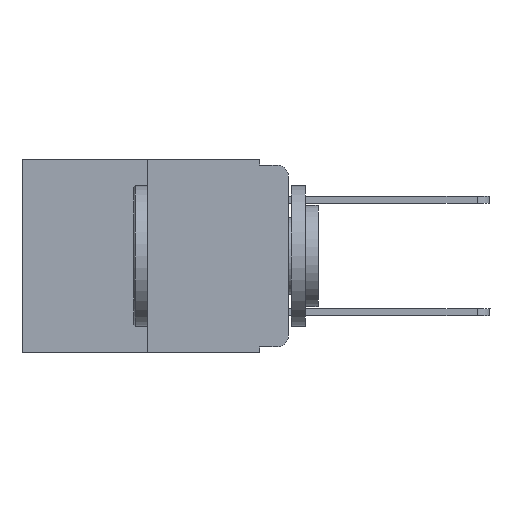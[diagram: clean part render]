
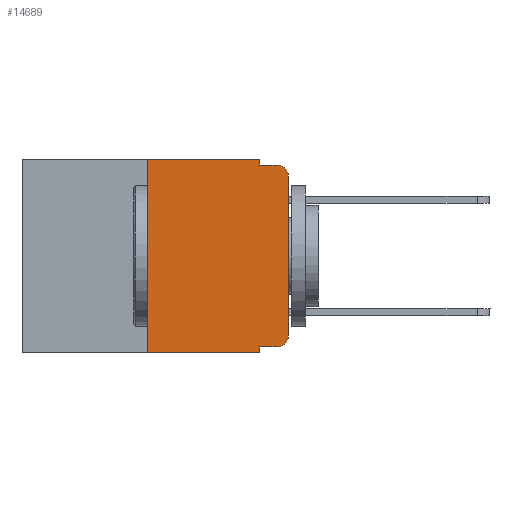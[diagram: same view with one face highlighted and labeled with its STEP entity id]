
A CAD part, left-side view. The second image highlights one B-rep face of the part: STEP entity #14689.
In plain terms, the highlighted planar face has unit normal (-1, 0, 0).
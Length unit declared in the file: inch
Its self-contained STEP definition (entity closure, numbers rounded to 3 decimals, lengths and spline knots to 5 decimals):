
#110 = DIRECTION ( 'NONE',  ( -1., 0., 0. ) ) ;
#189 = CARTESIAN_POINT ( 'NONE',  ( 0., 0.25, 0. ) ) ;
#237 = CARTESIAN_POINT ( 'NONE',  ( 0., 0.051, -0.333 ) ) ;
#295 = CARTESIAN_POINT ( 'NONE',  ( 0., 0.051, 0. ) ) ;
#404 = EDGE_CURVE ( 'NONE', #11798, #13101, #13912, .T. ) ;
#758 = ORIENTED_EDGE ( 'NONE', *, *, #7541, .T. ) ;
#784 = EDGE_CURVE ( 'NONE', #2574, #2361, #12662, .T. ) ;
#806 = EDGE_CURVE ( 'NONE', #6887, #14524, #15415, .T. ) ;
#812 = CARTESIAN_POINT ( 'NONE',  ( 0., 0., -0.313 ) ) ;
#875 = CARTESIAN_POINT ( 'NONE',  ( 0., 0., -0.03 ) ) ;
#1361 = EDGE_CURVE ( 'NONE', #11770, #13101, #15716, .T. ) ;
#1905 = ORIENTED_EDGE ( 'NONE', *, *, #8811, .F. ) ;
#1997 = CARTESIAN_POINT ( 'NONE',  ( 0., 0.473, -0.343 ) ) ;
#2109 = ORIENTED_EDGE ( 'NONE', *, *, #1361, .T. ) ;
#2127 = CARTESIAN_POINT ( 'NONE',  ( 0., 0.051, -0.333 ) ) ;
#2243 = LINE ( 'NONE', #4614, #11854 ) ;
#2361 = VERTEX_POINT ( 'NONE', #9852 ) ;
#2376 = CARTESIAN_POINT ( 'NONE',  ( 0., 0.051, 0. ) ) ;
#2535 = LINE ( 'NONE', #5153, #6289 ) ;
#2574 = VERTEX_POINT ( 'NONE', #189 ) ;
#2755 = DIRECTION ( 'NONE',  ( 0., -1., 0. ) ) ;
#2817 = DIRECTION ( 'NONE',  ( 0., 0., 1. ) ) ;
#2973 = AXIS2_PLACEMENT_3D ( 'NONE', #4204, #4367, #7921 ) ;
#3584 = LINE ( 'NONE', #2376, #13242 ) ;
#3916 = DIRECTION ( 'NONE',  ( 0., 0., -1. ) ) ;
#4102 = VECTOR ( 'NONE', #2755, 39.37008 ) ;
#4137 = VECTOR ( 'NONE', #5857, 39.37008 ) ;
#4204 = CARTESIAN_POINT ( 'NONE',  ( 0., 0.473, 0. ) ) ;
#4269 = CARTESIAN_POINT ( 'NONE',  ( 0., 0.051, -0.343 ) ) ;
#4367 = DIRECTION ( 'NONE',  ( 1., 0., 0. ) ) ;
#4370 = CIRCLE ( 'NONE', #14857, 0.02 ) ;
#4614 = CARTESIAN_POINT ( 'NONE',  ( 0., 0.051, -0.01 ) ) ;
#5028 = EDGE_CURVE ( 'NONE', #11826, #7764, #2243, .T. ) ;
#5089 = CARTESIAN_POINT ( 'NONE',  ( 0., 0.02, -0.03 ) ) ;
#5135 = LINE ( 'NONE', #237, #4102 ) ;
#5153 = CARTESIAN_POINT ( 'NONE',  ( 0., 0., 0. ) ) ;
#5310 = DIRECTION ( 'NONE',  ( 0., 0., 1. ) ) ;
#5428 = DIRECTION ( 'NONE',  ( 0., 0., -1. ) ) ;
#5498 = CARTESIAN_POINT ( 'NONE',  ( 0., 0.051, -0.01 ) ) ;
#5857 = DIRECTION ( 'NONE',  ( 0., -1., 0. ) ) ;
#6289 = VECTOR ( 'NONE', #5310, 39.37008 ) ;
#6387 = ORIENTED_EDGE ( 'NONE', *, *, #404, .F. ) ;
#6408 = ORIENTED_EDGE ( 'NONE', *, *, #15107, .F. ) ;
#6887 = VERTEX_POINT ( 'NONE', #7319 ) ;
#6968 = EDGE_CURVE ( 'NONE', #12727, #7764, #4370, .T. ) ;
#7319 = CARTESIAN_POINT ( 'NONE',  ( 0., 0.02, -0.333 ) ) ;
#7366 = CARTESIAN_POINT ( 'NONE',  ( 0., 0.02, -0.01 ) ) ;
#7541 = EDGE_CURVE ( 'NONE', #14524, #12727, #2535, .T. ) ;
#7764 = VERTEX_POINT ( 'NONE', #7366 ) ;
#7921 = DIRECTION ( 'NONE',  ( 0., 0., -1. ) ) ;
#8022 = CARTESIAN_POINT ( 'NONE',  ( 0., 0.02, -0.313 ) ) ;
#8543 = ORIENTED_EDGE ( 'NONE', *, *, #6968, .T. ) ;
#8811 = EDGE_CURVE ( 'NONE', #2361, #11826, #3584, .T. ) ;
#9339 = CARTESIAN_POINT ( 'NONE',  ( 0., 0.473, 0. ) ) ;
#9404 = FACE_OUTER_BOUND ( 'NONE', #14878, .T. ) ;
#9462 = EDGE_CURVE ( 'NONE', #11798, #6887, #5135, .T. ) ;
#9852 = CARTESIAN_POINT ( 'NONE',  ( 0., 0.051, 0. ) ) ;
#10184 = VECTOR ( 'NONE', #10565, 39.37008 ) ;
#10424 = AXIS2_PLACEMENT_3D ( 'NONE', #8022, #14267, #13971 ) ;
#10565 = DIRECTION ( 'NONE',  ( 0., -1., 0. ) ) ;
#11770 = VERTEX_POINT ( 'NONE', #11834 ) ;
#11798 = VERTEX_POINT ( 'NONE', #2127 ) ;
#11826 = VERTEX_POINT ( 'NONE', #5498 ) ;
#11834 = CARTESIAN_POINT ( 'NONE',  ( 0., 0.25, -0.343 ) ) ;
#11854 = VECTOR ( 'NONE', #13331, 39.37008 ) ;
#12662 = LINE ( 'NONE', #9339, #10184 ) ;
#12704 = VECTOR ( 'NONE', #2817, 39.37008 ) ;
#12727 = VERTEX_POINT ( 'NONE', #875 ) ;
#13101 = VERTEX_POINT ( 'NONE', #4269 ) ;
#13242 = VECTOR ( 'NONE', #3916, 39.37008 ) ;
#13331 = DIRECTION ( 'NONE',  ( 0., -1., 0. ) ) ;
#13912 = LINE ( 'NONE', #295, #15915 ) ;
#13954 = ORIENTED_EDGE ( 'NONE', *, *, #9462, .T. ) ;
#13968 = DIRECTION ( 'NONE',  ( 0., 0., -1. ) ) ;
#13971 = DIRECTION ( 'NONE',  ( 0., 0., -1. ) ) ;
#14144 = CARTESIAN_POINT ( 'NONE',  ( 0., 0.25, 0. ) ) ;
#14267 = DIRECTION ( 'NONE',  ( -1., 0., 0. ) ) ;
#14524 = VERTEX_POINT ( 'NONE', #812 ) ;
#14689 = ADVANCED_FACE ( 'NONE', ( #9404 ), #15630, .F. ) ;
#14773 = ORIENTED_EDGE ( 'NONE', *, *, #806, .T. ) ;
#14812 = ORIENTED_EDGE ( 'NONE', *, *, #784, .F. ) ;
#14857 = AXIS2_PLACEMENT_3D ( 'NONE', #5089, #110, #13968 ) ;
#14878 = EDGE_LOOP ( 'NONE', ( #758, #8543, #15734, #1905, #14812, #6408, #2109, #6387, #13954, #14773 ) ) ;
#15107 = EDGE_CURVE ( 'NONE', #11770, #2574, #16120, .T. ) ;
#15415 = CIRCLE ( 'NONE', #10424, 0.02 ) ;
#15630 = PLANE ( 'NONE',  #2973 ) ;
#15716 = LINE ( 'NONE', #1997, #4137 ) ;
#15734 = ORIENTED_EDGE ( 'NONE', *, *, #5028, .F. ) ;
#15915 = VECTOR ( 'NONE', #5428, 39.37008 ) ;
#16120 = LINE ( 'NONE', #14144, #12704 ) ;
